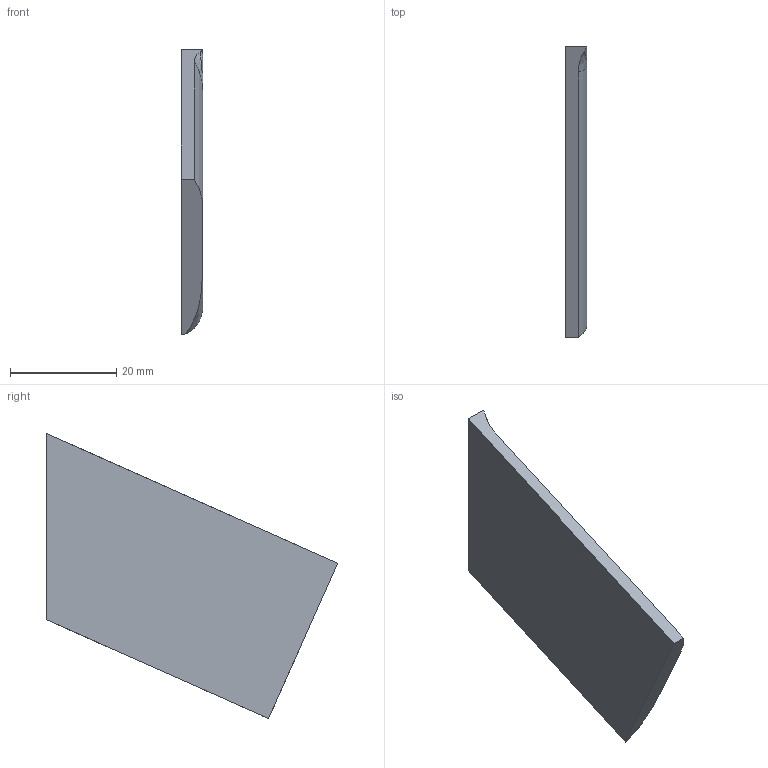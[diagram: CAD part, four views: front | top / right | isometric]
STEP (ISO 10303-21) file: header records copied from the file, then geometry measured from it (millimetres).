
FILE_DESCRIPTION((''),'2;1');
FILE_NAME('PM522GripPanel2.stp','2015-10-01T18:16:52',('JamesRPatrick'),(''),'Autodesk Inventor 2012','Autodesk Inventor 2012','');
FILE_SCHEMA(('AUTOMOTIVE_DESIGN { 1 0 10303 214 1 1 1 1 }'));
Length unit declared in the file: millimetre
Products named in the file (1): PM522GripPanel2
Bounding box: 4.1 x 54.81 x 53.64 mm (x, y, z)
Volume: 6723.8 mm3; surface area: 3987.1 mm2
Topology: 1 solids, 1 shells, 11 faces, 27 edges, 17 vertices
Faces by surface type: plane 6, bspline 4, cylinder 1
Entity records: 520 total; most frequent: CARTESIAN_POINT 260, ORIENTED_EDGE 52, DIRECTION 33, EDGE_CURVE 26, VERTEX_POINT 17, VECTOR 13, LINE 13, EDGE_LOOP 11
